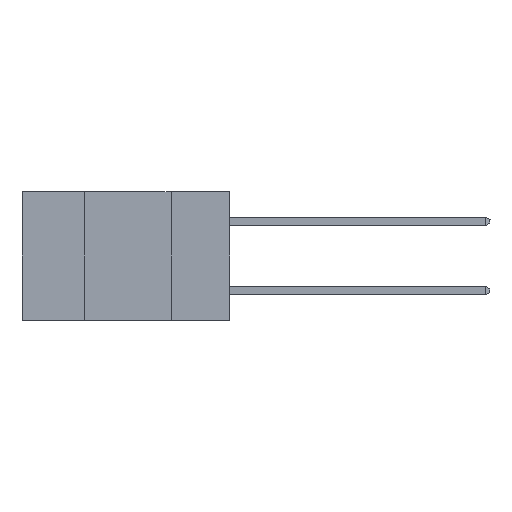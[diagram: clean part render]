
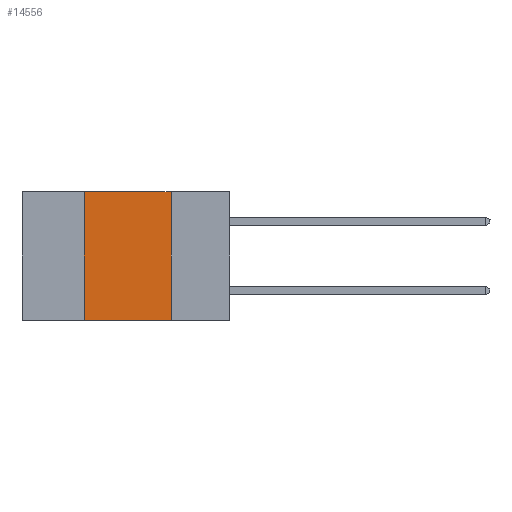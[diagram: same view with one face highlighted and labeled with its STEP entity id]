
A CAD part, left-side view. The second image highlights one B-rep face of the part: STEP entity #14556.
In plain terms, the highlighted planar face has unit normal (-1, 0, 0).
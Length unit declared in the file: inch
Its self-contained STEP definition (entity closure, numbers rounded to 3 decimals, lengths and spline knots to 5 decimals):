
#63 = ORIENTED_EDGE ( 'NONE', *, *, #7444, .F. ) ;
#388 = CARTESIAN_POINT ( 'NONE',  ( 0., 0.42, -0.37 ) ) ;
#684 = CARTESIAN_POINT ( 'NONE',  ( 0., 0.42, 0. ) ) ;
#4597 = EDGE_CURVE ( 'NONE', #13619, #13883, #10264, .T. ) ;
#4722 = VECTOR ( 'NONE', #8265, 39.37008 ) ;
#5247 = VECTOR ( 'NONE', #12938, 39.37008 ) ;
#6046 = DIRECTION ( 'NONE',  ( 1., 0., 0. ) ) ;
#6567 = DIRECTION ( 'NONE',  ( 0., 0., -1. ) ) ;
#7444 = EDGE_CURVE ( 'NONE', #11684, #13619, #8507, .T. ) ;
#8265 = DIRECTION ( 'NONE',  ( 0., -1., 0. ) ) ;
#8380 = FACE_OUTER_BOUND ( 'NONE', #16105, .T. ) ;
#8465 = CARTESIAN_POINT ( 'NONE',  ( 0., 0.6, 0. ) ) ;
#8507 = LINE ( 'NONE', #14842, #4722 ) ;
#8866 = EDGE_CURVE ( 'NONE', #10860, #11684, #10601, .T. ) ;
#8999 = CARTESIAN_POINT ( 'NONE',  ( 0., 0.42, 0. ) ) ;
#9235 = CARTESIAN_POINT ( 'NONE',  ( 0., 0.17, 0. ) ) ;
#9804 = DIRECTION ( 'NONE',  ( 0., 0., -1. ) ) ;
#10233 = EDGE_CURVE ( 'NONE', #10860, #13883, #13855, .T. ) ;
#10264 = LINE ( 'NONE', #9235, #15880 ) ;
#10601 = LINE ( 'NONE', #8999, #5247 ) ;
#10860 = VERTEX_POINT ( 'NONE', #388 ) ;
#11327 = VECTOR ( 'NONE', #15508, 39.37008 ) ;
#11684 = VERTEX_POINT ( 'NONE', #684 ) ;
#11952 = ORIENTED_EDGE ( 'NONE', *, *, #8866, .F. ) ;
#12909 = CARTESIAN_POINT ( 'NONE',  ( 0., 0.6, -0.37 ) ) ;
#12938 = DIRECTION ( 'NONE',  ( 0., 0., 1. ) ) ;
#13453 = ORIENTED_EDGE ( 'NONE', *, *, #4597, .F. ) ;
#13619 = VERTEX_POINT ( 'NONE', #16042 ) ;
#13855 = LINE ( 'NONE', #12909, #11327 ) ;
#13883 = VERTEX_POINT ( 'NONE', #14800 ) ;
#14259 = AXIS2_PLACEMENT_3D ( 'NONE', #8465, #6046, #9804 ) ;
#14556 = ADVANCED_FACE ( 'NONE', ( #8380 ), #16014, .F. ) ;
#14724 = ORIENTED_EDGE ( 'NONE', *, *, #10233, .T. ) ;
#14800 = CARTESIAN_POINT ( 'NONE',  ( 0., 0.17, -0.37 ) ) ;
#14842 = CARTESIAN_POINT ( 'NONE',  ( 0., 0.6, 0. ) ) ;
#15508 = DIRECTION ( 'NONE',  ( 0., -1., 0. ) ) ;
#15880 = VECTOR ( 'NONE', #6567, 39.37008 ) ;
#16014 = PLANE ( 'NONE',  #14259 ) ;
#16042 = CARTESIAN_POINT ( 'NONE',  ( 0., 0.17, 0. ) ) ;
#16105 = EDGE_LOOP ( 'NONE', ( #13453, #63, #11952, #14724 ) ) ;
